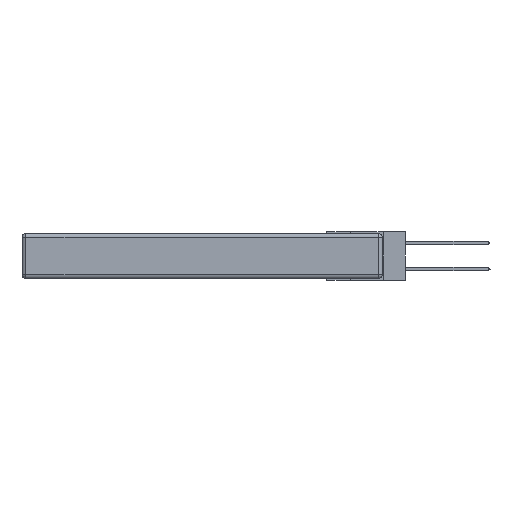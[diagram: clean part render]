
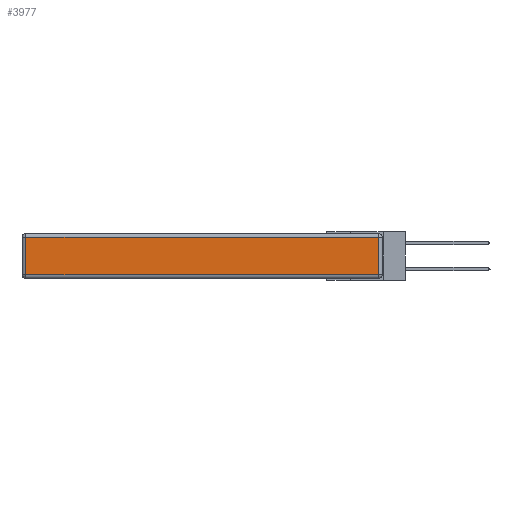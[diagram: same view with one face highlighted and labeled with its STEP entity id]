
A CAD part, left-side view. The second image highlights one B-rep face of the part: STEP entity #3977.
In plain terms, the highlighted planar face has unit normal (-1, 0, 0).
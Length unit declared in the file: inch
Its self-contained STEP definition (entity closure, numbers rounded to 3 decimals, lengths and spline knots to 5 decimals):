
#625 = VERTEX_POINT ( 'NONE', #4605 ) ;
#1214 = ORIENTED_EDGE ( 'NONE', *, *, #1735, .T. ) ;
#1735 = EDGE_CURVE ( 'NONE', #12049, #5215, #18931, .T. ) ;
#1755 = EDGE_LOOP ( 'NONE', ( #4817, #1214, #4108, #12638 ) ) ;
#2929 = VECTOR ( 'NONE', #4535, 39.37008 ) ;
#3977 = ADVANCED_FACE ( 'NONE', ( #10267 ), #16744, .T. ) ;
#4108 = ORIENTED_EDGE ( 'NONE', *, *, #11654, .T. ) ;
#4221 = VECTOR ( 'NONE', #16102, 39.37008 ) ;
#4535 = DIRECTION ( 'NONE',  ( 0., 0., 1. ) ) ;
#4605 = CARTESIAN_POINT ( 'NONE',  ( 0., 2.72, -0.03 ) ) ;
#4817 = ORIENTED_EDGE ( 'NONE', *, *, #26075, .T. ) ;
#5215 = VERTEX_POINT ( 'NONE', #14404 ) ;
#6515 = CARTESIAN_POINT ( 'NONE',  ( 0., 0., -0.343 ) ) ;
#7298 = DIRECTION ( 'NONE',  ( 0., 0., -1. ) ) ;
#10267 = FACE_OUTER_BOUND ( 'NONE', #1755, .T. ) ;
#10802 = VECTOR ( 'NONE', #22611, 39.37008 ) ;
#11654 = EDGE_CURVE ( 'NONE', #5215, #625, #18903, .T. ) ;
#12049 = VERTEX_POINT ( 'NONE', #20193 ) ;
#12638 = ORIENTED_EDGE ( 'NONE', *, *, #18013, .T. ) ;
#12715 = DIRECTION ( 'NONE',  ( -1., 0., 0. ) ) ;
#12957 = CARTESIAN_POINT ( 'NONE',  ( 0., 2.72, -0.343 ) ) ;
#12997 = CARTESIAN_POINT ( 'NONE',  ( 0., 2.72, -0.313 ) ) ;
#14185 = AXIS2_PLACEMENT_3D ( 'NONE', #6515, #12715, #25300 ) ;
#14229 = VERTEX_POINT ( 'NONE', #12997 ) ;
#14404 = CARTESIAN_POINT ( 'NONE',  ( 0., 0.03, -0.03 ) ) ;
#16102 = DIRECTION ( 'NONE',  ( 0., 1., 0. ) ) ;
#16270 = CARTESIAN_POINT ( 'NONE',  ( 0., 0., -0.313 ) ) ;
#16388 = LINE ( 'NONE', #16270, #10802 ) ;
#16744 = PLANE ( 'NONE',  #14185 ) ;
#17462 = VECTOR ( 'NONE', #7298, 39.37008 ) ;
#18013 = EDGE_CURVE ( 'NONE', #625, #14229, #23032, .T. ) ;
#18903 = LINE ( 'NONE', #24308, #4221 ) ;
#18931 = LINE ( 'NONE', #27019, #2929 ) ;
#20193 = CARTESIAN_POINT ( 'NONE',  ( 0., 0.03, -0.313 ) ) ;
#22611 = DIRECTION ( 'NONE',  ( 0., -1., 0. ) ) ;
#23032 = LINE ( 'NONE', #12957, #17462 ) ;
#24308 = CARTESIAN_POINT ( 'NONE',  ( 0., 2.75, -0.03 ) ) ;
#25300 = DIRECTION ( 'NONE',  ( 0., 0., 1. ) ) ;
#26075 = EDGE_CURVE ( 'NONE', #14229, #12049, #16388, .T. ) ;
#27019 = CARTESIAN_POINT ( 'NONE',  ( 0., 0.03, -0.343 ) ) ;
